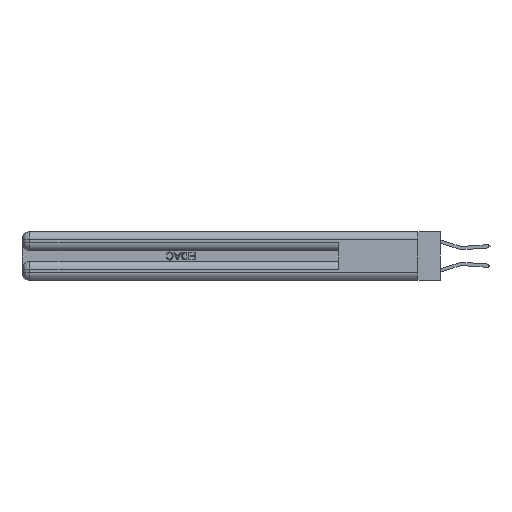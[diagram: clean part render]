
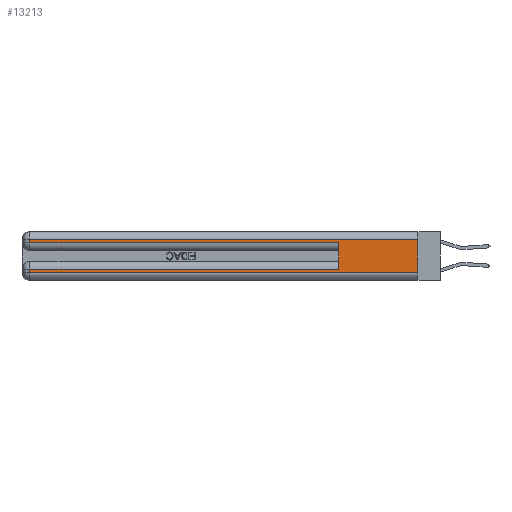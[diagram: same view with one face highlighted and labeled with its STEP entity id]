
A CAD part, left-side view. The second image highlights one B-rep face of the part: STEP entity #13213.
In plain terms, the highlighted planar face has unit normal (-1, 0, 0).
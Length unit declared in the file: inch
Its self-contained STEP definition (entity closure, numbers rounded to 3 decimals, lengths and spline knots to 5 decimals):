
#194 = VERTEX_POINT ( 'NONE', #3407 ) ;
#342 = LINE ( 'NONE', #11228, #6631 ) ;
#420 = CARTESIAN_POINT ( 'NONE',  ( 0., 0., 0.085 ) ) ;
#556 = DIRECTION ( 'NONE',  ( 0., 0., -1. ) ) ;
#868 = DIRECTION ( 'NONE',  ( 0., 1., 0. ) ) ;
#2215 = AXIS2_PLACEMENT_3D ( 'NONE', #30596, #14779, #33228 ) ;
#2488 = ORIENTED_EDGE ( 'NONE', *, *, #20715, .F. ) ;
#2744 = VECTOR ( 'NONE', #19236, 39.37008 ) ;
#3407 = CARTESIAN_POINT ( 'NONE',  ( 0., 0.6, 0.085 ) ) ;
#4441 = CARTESIAN_POINT ( 'NONE',  ( 0., 2.94, 0.285 ) ) ;
#5011 = EDGE_CURVE ( 'NONE', #30756, #23500, #5257, .T. ) ;
#5257 = LINE ( 'NONE', #24554, #2744 ) ;
#5870 = ORIENTED_EDGE ( 'NONE', *, *, #27088, .T. ) ;
#5905 = CARTESIAN_POINT ( 'NONE',  ( 0., 0., 0.285 ) ) ;
#6188 = VECTOR ( 'NONE', #868, 39.37008 ) ;
#6631 = VECTOR ( 'NONE', #556, 39.37008 ) ;
#7062 = CARTESIAN_POINT ( 'NONE',  ( 0., 2.94, 0.31 ) ) ;
#7610 = EDGE_LOOP ( 'NONE', ( #32333, #26664, #7902, #5870, #2488, #20955, #13979, #28855 ) ) ;
#7902 = ORIENTED_EDGE ( 'NONE', *, *, #5011, .T. ) ;
#8602 = DIRECTION ( 'NONE',  ( 0., -1., 0. ) ) ;
#8972 = CARTESIAN_POINT ( 'NONE',  ( 0., 0., 0.06 ) ) ;
#9729 = DIRECTION ( 'NONE',  ( 0., 0., -1. ) ) ;
#10234 = EDGE_CURVE ( 'NONE', #20694, #26524, #342, .T. ) ;
#10313 = VECTOR ( 'NONE', #9729, 39.37008 ) ;
#10570 = CARTESIAN_POINT ( 'NONE',  ( 0., 0.6, 0.145 ) ) ;
#11101 = CARTESIAN_POINT ( 'NONE',  ( 0., 0., 0.31 ) ) ;
#11191 = VERTEX_POINT ( 'NONE', #17207 ) ;
#11228 = CARTESIAN_POINT ( 'NONE',  ( 0., 2.94, 0.37 ) ) ;
#12085 = PLANE ( 'NONE',  #2215 ) ;
#13213 = ADVANCED_FACE ( 'NONE', ( #30460 ), #12085, .F. ) ;
#13277 = DIRECTION ( 'NONE',  ( 0., 0., 1. ) ) ;
#13979 = ORIENTED_EDGE ( 'NONE', *, *, #10234, .T. ) ;
#14779 = DIRECTION ( 'NONE',  ( 1., 0., 0. ) ) ;
#15827 = CARTESIAN_POINT ( 'NONE',  ( 0., 2.94, 0.085 ) ) ;
#15859 = VERTEX_POINT ( 'NONE', #11101 ) ;
#16056 = VECTOR ( 'NONE', #22229, 39.37008 ) ;
#17207 = CARTESIAN_POINT ( 'NONE',  ( 0., 0., 0.06 ) ) ;
#18538 = VECTOR ( 'NONE', #13277, 39.37008 ) ;
#19236 = DIRECTION ( 'NONE',  ( 0., 0., -1. ) ) ;
#20063 = VECTOR ( 'NONE', #8602, 39.37008 ) ;
#20220 = EDGE_CURVE ( 'NONE', #194, #20694, #27260, .T. ) ;
#20222 = VECTOR ( 'NONE', #29741, 39.37008 ) ;
#20328 = EDGE_CURVE ( 'NONE', #26524, #11191, #23111, .T. ) ;
#20694 = VERTEX_POINT ( 'NONE', #15827 ) ;
#20715 = EDGE_CURVE ( 'NONE', #194, #22278, #32562, .T. ) ;
#20955 = ORIENTED_EDGE ( 'NONE', *, *, #20220, .T. ) ;
#22229 = DIRECTION ( 'NONE',  ( 0., -1., 0. ) ) ;
#22278 = VERTEX_POINT ( 'NONE', #22696 ) ;
#22696 = CARTESIAN_POINT ( 'NONE',  ( 0., 0.6, 0.285 ) ) ;
#23111 = LINE ( 'NONE', #8972, #16056 ) ;
#23500 = VERTEX_POINT ( 'NONE', #4441 ) ;
#24554 = CARTESIAN_POINT ( 'NONE',  ( 0., 2.94, 0.37 ) ) ;
#25644 = CARTESIAN_POINT ( 'NONE',  ( 0., 0., 0.37 ) ) ;
#26524 = VERTEX_POINT ( 'NONE', #30096 ) ;
#26664 = ORIENTED_EDGE ( 'NONE', *, *, #33369, .T. ) ;
#27088 = EDGE_CURVE ( 'NONE', #23500, #22278, #34064, .T. ) ;
#27260 = LINE ( 'NONE', #420, #20222 ) ;
#28855 = ORIENTED_EDGE ( 'NONE', *, *, #20328, .T. ) ;
#29741 = DIRECTION ( 'NONE',  ( 0., 1., 0. ) ) ;
#30096 = CARTESIAN_POINT ( 'NONE',  ( 0., 2.94, 0.06 ) ) ;
#30460 = FACE_OUTER_BOUND ( 'NONE', #7610, .T. ) ;
#30596 = CARTESIAN_POINT ( 'NONE',  ( 0., 0., 0.37 ) ) ;
#30614 = LINE ( 'NONE', #25644, #10313 ) ;
#30756 = VERTEX_POINT ( 'NONE', #7062 ) ;
#32333 = ORIENTED_EDGE ( 'NONE', *, *, #34169, .F. ) ;
#32562 = LINE ( 'NONE', #10570, #18538 ) ;
#32701 = CARTESIAN_POINT ( 'NONE',  ( 0., 0., 0.31 ) ) ;
#33228 = DIRECTION ( 'NONE',  ( 0., 0., -1. ) ) ;
#33369 = EDGE_CURVE ( 'NONE', #15859, #30756, #33545, .T. ) ;
#33545 = LINE ( 'NONE', #32701, #6188 ) ;
#34064 = LINE ( 'NONE', #5905, #20063 ) ;
#34169 = EDGE_CURVE ( 'NONE', #15859, #11191, #30614, .T. ) ;
